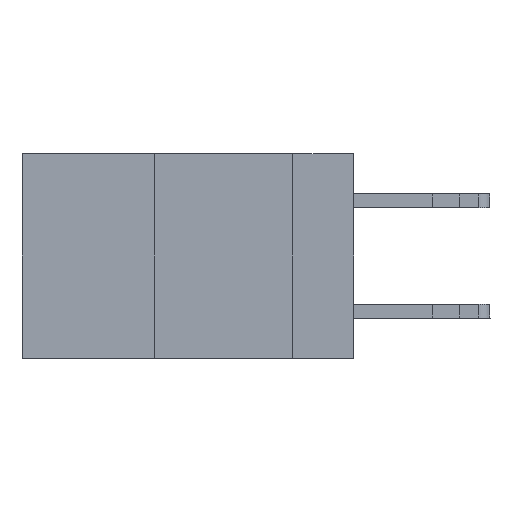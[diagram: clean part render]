
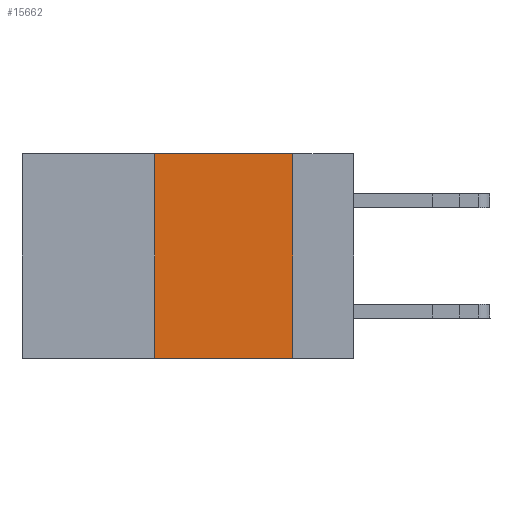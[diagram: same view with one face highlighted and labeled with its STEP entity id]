
A CAD part, left-side view. The second image highlights one B-rep face of the part: STEP entity #15662.
In plain terms, the highlighted planar face has unit normal (-1, 0, 0).
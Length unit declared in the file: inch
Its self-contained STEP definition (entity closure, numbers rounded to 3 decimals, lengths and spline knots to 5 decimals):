
#98 = CARTESIAN_POINT ( 'NONE',  ( 0., 0.36, -0.37 ) ) ;
#1597 = EDGE_CURVE ( 'NONE', #20811, #17903, #23005, .T. ) ;
#2821 = CARTESIAN_POINT ( 'NONE',  ( 0., 0.11, 0. ) ) ;
#2975 = EDGE_CURVE ( 'NONE', #17844, #17903, #15545, .T. ) ;
#3026 = DIRECTION ( 'NONE',  ( 0., 0., -1. ) ) ;
#6273 = CARTESIAN_POINT ( 'NONE',  ( 0., 0.6, 0. ) ) ;
#8089 = DIRECTION ( 'NONE',  ( 0., -1., 0. ) ) ;
#8483 = VECTOR ( 'NONE', #19821, 39.37008 ) ;
#9077 = CARTESIAN_POINT ( 'NONE',  ( 0., 0.36, 0. ) ) ;
#9494 = PLANE ( 'NONE',  #10885 ) ;
#10193 = VECTOR ( 'NONE', #3026, 39.37008 ) ;
#10885 = AXIS2_PLACEMENT_3D ( 'NONE', #16674, #21941, #11345 ) ;
#11345 = DIRECTION ( 'NONE',  ( 0., 0., -1. ) ) ;
#12982 = EDGE_CURVE ( 'NONE', #20811, #13628, #13365, .T. ) ;
#13365 = LINE ( 'NONE', #18063, #8483 ) ;
#13628 = VERTEX_POINT ( 'NONE', #9077 ) ;
#13677 = VECTOR ( 'NONE', #20808, 39.37008 ) ;
#14605 = LINE ( 'NONE', #6273, #22840 ) ;
#15273 = CARTESIAN_POINT ( 'NONE',  ( 0., 0.6, -0.37 ) ) ;
#15545 = LINE ( 'NONE', #2821, #10193 ) ;
#15662 = ADVANCED_FACE ( 'NONE', ( #22579 ), #9494, .F. ) ;
#15822 = EDGE_CURVE ( 'NONE', #13628, #17844, #14605, .T. ) ;
#16674 = CARTESIAN_POINT ( 'NONE',  ( 0., 0.6, 0. ) ) ;
#17577 = ORIENTED_EDGE ( 'NONE', *, *, #12982, .F. ) ;
#17844 = VERTEX_POINT ( 'NONE', #20602 ) ;
#17903 = VERTEX_POINT ( 'NONE', #20754 ) ;
#18063 = CARTESIAN_POINT ( 'NONE',  ( 0., 0.36, 0. ) ) ;
#18365 = ORIENTED_EDGE ( 'NONE', *, *, #15822, .F. ) ;
#19416 = EDGE_LOOP ( 'NONE', ( #21373, #18365, #17577, #19454 ) ) ;
#19454 = ORIENTED_EDGE ( 'NONE', *, *, #1597, .T. ) ;
#19821 = DIRECTION ( 'NONE',  ( 0., 0., 1. ) ) ;
#20602 = CARTESIAN_POINT ( 'NONE',  ( 0., 0.11, 0. ) ) ;
#20754 = CARTESIAN_POINT ( 'NONE',  ( 0., 0.11, -0.37 ) ) ;
#20808 = DIRECTION ( 'NONE',  ( 0., -1., 0. ) ) ;
#20811 = VERTEX_POINT ( 'NONE', #98 ) ;
#21373 = ORIENTED_EDGE ( 'NONE', *, *, #2975, .F. ) ;
#21941 = DIRECTION ( 'NONE',  ( 1., 0., 0. ) ) ;
#22579 = FACE_OUTER_BOUND ( 'NONE', #19416, .T. ) ;
#22840 = VECTOR ( 'NONE', #8089, 39.37008 ) ;
#23005 = LINE ( 'NONE', #15273, #13677 ) ;
